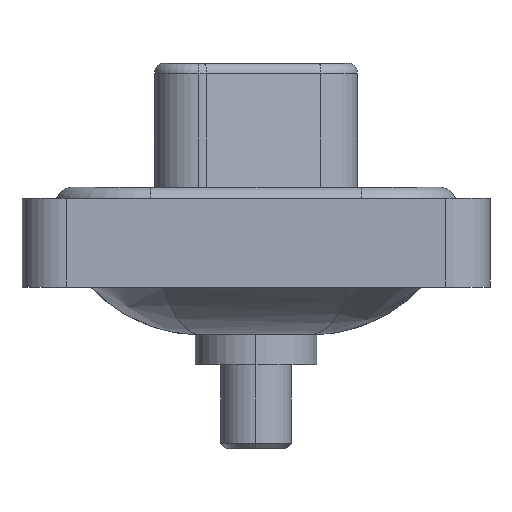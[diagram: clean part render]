
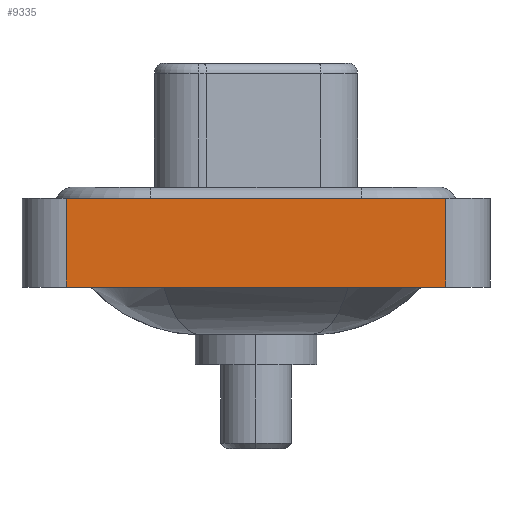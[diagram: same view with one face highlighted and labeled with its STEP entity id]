
A CAD part, left-side view. The second image highlights one B-rep face of the part: STEP entity #9335.
In plain terms, the highlighted planar face has unit normal (-1, 0, 0).
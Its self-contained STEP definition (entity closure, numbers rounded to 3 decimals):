
#37 = ORIENTED_EDGE ( 'NONE', *, *, #19047, .F. ) ;
#55 = VECTOR ( 'NONE', #9573, 1000. ) ;
#505 = LINE ( 'NONE', #6402, #55 ) ;
#937 = VERTEX_POINT ( 'NONE', #6533 ) ;
#1304 = VECTOR ( 'NONE', #2381, 1000. ) ;
#1679 = VERTEX_POINT ( 'NONE', #8063 ) ;
#2381 = DIRECTION ( 'NONE',  ( 0., -1., 0. ) ) ;
#2759 = LINE ( 'NONE', #6915, #1304 ) ;
#2974 = CARTESIAN_POINT ( 'NONE',  ( -7.3, -8.55, -3.6 ) ) ;
#3059 = DIRECTION ( 'NONE',  ( 0., 0., 1. ) ) ;
#4483 = DIRECTION ( 'NONE',  ( 0., 0., 1. ) ) ;
#5288 = AXIS2_PLACEMENT_3D ( 'NONE', #2974, #13504, #3059 ) ;
#5757 = EDGE_CURVE ( 'NONE', #16417, #15331, #12062, .T. ) ;
#5975 = VECTOR ( 'NONE', #13830, 1000. ) ;
#6402 = CARTESIAN_POINT ( 'NONE',  ( -7.3, -8.55, -3.6 ) ) ;
#6533 = CARTESIAN_POINT ( 'NONE',  ( -7.3, -8.55, -3.6 ) ) ;
#6915 = CARTESIAN_POINT ( 'NONE',  ( -7.3, -8.55, -3.6 ) ) ;
#8063 = CARTESIAN_POINT ( 'NONE',  ( -7.3, 8.55, -3.6 ) ) ;
#8743 = ORIENTED_EDGE ( 'NONE', *, *, #13914, .T. ) ;
#8854 = VECTOR ( 'NONE', #4483, 1000. ) ;
#9335 = ADVANCED_FACE ( 'NONE', ( #17558 ), #17840, .T. ) ;
#9421 = CARTESIAN_POINT ( 'NONE',  ( -7.3, -8.55, 0.4 ) ) ;
#9573 = DIRECTION ( 'NONE',  ( 0., 0., 1. ) ) ;
#9955 = CARTESIAN_POINT ( 'NONE',  ( -7.3, 8.55, 0.4 ) ) ;
#11676 = EDGE_LOOP ( 'NONE', ( #8743, #13088, #37, #17486 ) ) ;
#12062 = LINE ( 'NONE', #17877, #5975 ) ;
#13088 = ORIENTED_EDGE ( 'NONE', *, *, #5757, .F. ) ;
#13472 = LINE ( 'NONE', #17985, #8854 ) ;
#13504 = DIRECTION ( 'NONE',  ( -1., 0., 0. ) ) ;
#13830 = DIRECTION ( 'NONE',  ( 0., -1., 0. ) ) ;
#13914 = EDGE_CURVE ( 'NONE', #937, #15331, #505, .T. ) ;
#15331 = VERTEX_POINT ( 'NONE', #9421 ) ;
#16417 = VERTEX_POINT ( 'NONE', #9955 ) ;
#17328 = EDGE_CURVE ( 'NONE', #1679, #937, #2759, .T. ) ;
#17486 = ORIENTED_EDGE ( 'NONE', *, *, #17328, .T. ) ;
#17558 = FACE_OUTER_BOUND ( 'NONE', #11676, .T. ) ;
#17840 = PLANE ( 'NONE',  #5288 ) ;
#17877 = CARTESIAN_POINT ( 'NONE',  ( -7.3, -8.55, 0.4 ) ) ;
#17985 = CARTESIAN_POINT ( 'NONE',  ( -7.3, 8.55, -3.6 ) ) ;
#19047 = EDGE_CURVE ( 'NONE', #1679, #16417, #13472, .T. ) ;
